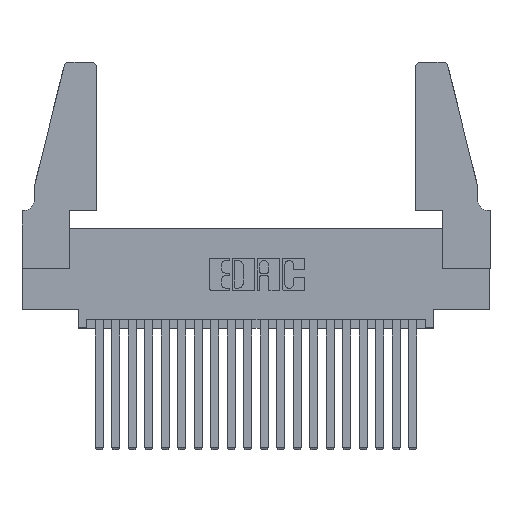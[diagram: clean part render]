
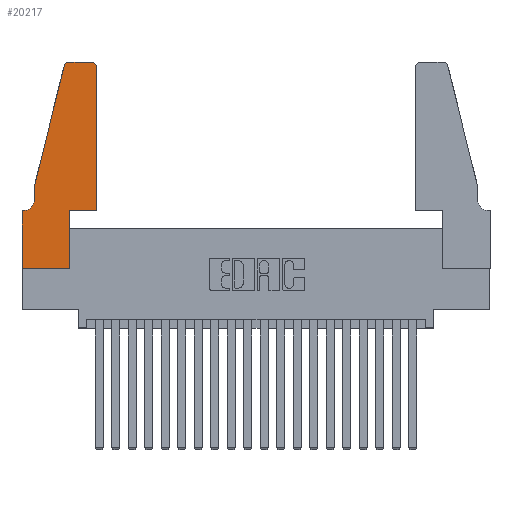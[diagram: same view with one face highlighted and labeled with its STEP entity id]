
A CAD part, top view. The second image highlights one B-rep face of the part: STEP entity #20217.
In plain terms, the highlighted planar face has unit normal (0, 0, 1).
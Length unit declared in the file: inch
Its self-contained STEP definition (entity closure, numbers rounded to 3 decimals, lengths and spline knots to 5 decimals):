
#63 = CIRCLE ( 'NONE', #4833, 0.03 ) ;
#71 = VECTOR ( 'NONE', #2145, 39.37008 ) ;
#83 = VECTOR ( 'NONE', #9493, 39.37008 ) ;
#277 = CARTESIAN_POINT ( 'NONE',  ( 0.2865, 0.35, 0.37 ) ) ;
#916 = ORIENTED_EDGE ( 'NONE', *, *, #2555, .T. ) ;
#964 = DIRECTION ( 'NONE',  ( 1., 0., 0. ) ) ;
#1077 = CARTESIAN_POINT ( 'NONE',  ( 0., 0., 0.37 ) ) ;
#1132 = EDGE_CURVE ( 'NONE', #18445, #18649, #6520, .T. ) ;
#1245 = CARTESIAN_POINT ( 'NONE',  ( 0.0755, 0.5, 0.37 ) ) ;
#1249 = VERTEX_POINT ( 'NONE', #6440 ) ;
#1459 = ORIENTED_EDGE ( 'NONE', *, *, #18032, .T. ) ;
#1578 = CIRCLE ( 'NONE', #18708, 0.03 ) ;
#1584 = CARTESIAN_POINT ( 'NONE',  ( 0., 0.35, 0.37 ) ) ;
#1736 = ORIENTED_EDGE ( 'NONE', *, *, #1132, .T. ) ;
#2145 = DIRECTION ( 'NONE',  ( 0., -1., 0. ) ) ;
#2345 = ORIENTED_EDGE ( 'NONE', *, *, #17151, .T. ) ;
#2362 = ORIENTED_EDGE ( 'NONE', *, *, #14664, .T. ) ;
#2456 = EDGE_CURVE ( 'NONE', #7041, #6586, #6937, .T. ) ;
#2555 = EDGE_CURVE ( 'NONE', #18649, #19597, #6683, .T. ) ;
#2651 = VERTEX_POINT ( 'NONE', #14811 ) ;
#3199 = CARTESIAN_POINT ( 'NONE',  ( 0.4205, 1.22, 0.37 ) ) ;
#3210 = DIRECTION ( 'NONE',  ( 0., 0., 1. ) ) ;
#3926 = EDGE_CURVE ( 'NONE', #1249, #4341, #18651, .T. ) ;
#4341 = VERTEX_POINT ( 'NONE', #12725 ) ;
#4622 = CARTESIAN_POINT ( 'NONE',  ( 0.2605, 1.25, 0.37 ) ) ;
#4833 = AXIS2_PLACEMENT_3D ( 'NONE', #5754, #20140, #964 ) ;
#5385 = ORIENTED_EDGE ( 'NONE', *, *, #16853, .T. ) ;
#5754 = CARTESIAN_POINT ( 'NONE',  ( 0.284, 1.22, 0.37 ) ) ;
#5901 = LINE ( 'NONE', #9222, #13915 ) ;
#6440 = CARTESIAN_POINT ( 'NONE',  ( 0.4205, 1.25, 0.37 ) ) ;
#6520 = LINE ( 'NONE', #1077, #14517 ) ;
#6586 = VERTEX_POINT ( 'NONE', #14233 ) ;
#6683 = LINE ( 'NONE', #9664, #11425 ) ;
#6937 = LINE ( 'NONE', #1245, #18170 ) ;
#6980 = EDGE_CURVE ( 'NONE', #19597, #17285, #10167, .T. ) ;
#7041 = VERTEX_POINT ( 'NONE', #12010 ) ;
#7139 = VECTOR ( 'NONE', #19183, 39.37008 ) ;
#7162 = LINE ( 'NONE', #14530, #8411 ) ;
#7263 = CARTESIAN_POINT ( 'NONE',  ( 0.4505, 0.35, 0.37 ) ) ;
#7593 = DIRECTION ( 'NONE',  ( -0.239, -0.971, 0. ) ) ;
#7916 = PLANE ( 'NONE',  #12781 ) ;
#7977 = EDGE_CURVE ( 'NONE', #9011, #1249, #1578, .T. ) ;
#7987 = CARTESIAN_POINT ( 'NONE',  ( 0.0055, 0.35, 0.37 ) ) ;
#8018 = ORIENTED_EDGE ( 'NONE', *, *, #17773, .T. ) ;
#8166 = DIRECTION ( 'NONE',  ( -1., 0., 0. ) ) ;
#8326 = AXIS2_PLACEMENT_3D ( 'NONE', #14010, #18814, #10862 ) ;
#8411 = VECTOR ( 'NONE', #8166, 39.37008 ) ;
#8809 = CARTESIAN_POINT ( 'NONE',  ( 0.4505, 0.35, 0.37 ) ) ;
#8859 = LINE ( 'NONE', #19618, #83 ) ;
#9011 = VERTEX_POINT ( 'NONE', #18805 ) ;
#9222 = CARTESIAN_POINT ( 'NONE',  ( 0.0755, 0.5, 0.37 ) ) ;
#9230 = ORIENTED_EDGE ( 'NONE', *, *, #7977, .T. ) ;
#9253 = ORIENTED_EDGE ( 'NONE', *, *, #2456, .T. ) ;
#9493 = DIRECTION ( 'NONE',  ( 0., 1., 0. ) ) ;
#9664 = CARTESIAN_POINT ( 'NONE',  ( 0.2865, 0.35, 0.37 ) ) ;
#10167 = LINE ( 'NONE', #8809, #11412 ) ;
#10442 = ORIENTED_EDGE ( 'NONE', *, *, #3926, .T. ) ;
#10549 = EDGE_LOOP ( 'NONE', ( #10442, #2345, #20662, #9253, #1459, #2362, #8018, #1736, #916, #19203, #5385, #9230 ) ) ;
#10594 = CARTESIAN_POINT ( 'NONE',  ( 0.25487, 1.22718, 0.37 ) ) ;
#10862 = DIRECTION ( 'NONE',  ( -1., 0., 0. ) ) ;
#11412 = VECTOR ( 'NONE', #13628, 39.37008 ) ;
#11425 = VECTOR ( 'NONE', #19174, 39.37008 ) ;
#12010 = CARTESIAN_POINT ( 'NONE',  ( 0.0755, 0.5, 0.37 ) ) ;
#12725 = CARTESIAN_POINT ( 'NONE',  ( 0.284, 1.25, 0.37 ) ) ;
#12781 = AXIS2_PLACEMENT_3D ( 'NONE', #1584, #3210, #14420 ) ;
#13628 = DIRECTION ( 'NONE',  ( 1., 0., 0. ) ) ;
#13915 = VECTOR ( 'NONE', #7593, 39.37008 ) ;
#14004 = VERTEX_POINT ( 'NONE', #7987 ) ;
#14010 = CARTESIAN_POINT ( 'NONE',  ( 0.0055, 0.42, 0.37 ) ) ;
#14073 = DIRECTION ( 'NONE',  ( 0., -1., 0. ) ) ;
#14119 = DIRECTION ( 'NONE',  ( 1., 0., 0. ) ) ;
#14233 = CARTESIAN_POINT ( 'NONE',  ( 0.0755, 0.42, 0.37 ) ) ;
#14420 = DIRECTION ( 'NONE',  ( 1., 0., 0. ) ) ;
#14502 = FACE_OUTER_BOUND ( 'NONE', #10549, .T. ) ;
#14517 = VECTOR ( 'NONE', #14119, 39.37008 ) ;
#14530 = CARTESIAN_POINT ( 'NONE',  ( 0.0755, 0.35, 0.37 ) ) ;
#14664 = EDGE_CURVE ( 'NONE', #14004, #2651, #7162, .T. ) ;
#14811 = CARTESIAN_POINT ( 'NONE',  ( 0., 0.35, 0.37 ) ) ;
#15195 = EDGE_CURVE ( 'NONE', #18552, #7041, #5901, .T. ) ;
#15507 = CARTESIAN_POINT ( 'NONE',  ( 0.2865, 0., 0.37 ) ) ;
#15870 = DIRECTION ( 'NONE',  ( 0., 0., 1. ) ) ;
#16853 = EDGE_CURVE ( 'NONE', #17285, #9011, #8859, .T. ) ;
#17151 = EDGE_CURVE ( 'NONE', #4341, #18552, #63, .T. ) ;
#17285 = VERTEX_POINT ( 'NONE', #7263 ) ;
#17587 = DIRECTION ( 'NONE',  ( 1., 0., 0. ) ) ;
#17696 = CARTESIAN_POINT ( 'NONE',  ( 0., 0., 0.37 ) ) ;
#17773 = EDGE_CURVE ( 'NONE', #2651, #18445, #18063, .T. ) ;
#18032 = EDGE_CURVE ( 'NONE', #6586, #14004, #18043, .T. ) ;
#18043 = CIRCLE ( 'NONE', #8326, 0.07 ) ;
#18063 = LINE ( 'NONE', #18831, #71 ) ;
#18170 = VECTOR ( 'NONE', #14073, 39.37008 ) ;
#18445 = VERTEX_POINT ( 'NONE', #17696 ) ;
#18552 = VERTEX_POINT ( 'NONE', #10594 ) ;
#18649 = VERTEX_POINT ( 'NONE', #15507 ) ;
#18651 = LINE ( 'NONE', #4622, #7139 ) ;
#18708 = AXIS2_PLACEMENT_3D ( 'NONE', #3199, #15870, #17587 ) ;
#18805 = CARTESIAN_POINT ( 'NONE',  ( 0.4505, 1.22, 0.37 ) ) ;
#18814 = DIRECTION ( 'NONE',  ( 0., 0., -1. ) ) ;
#18831 = CARTESIAN_POINT ( 'NONE',  ( 0., 0., 0.37 ) ) ;
#19174 = DIRECTION ( 'NONE',  ( 0., 1., 0. ) ) ;
#19183 = DIRECTION ( 'NONE',  ( -1., 0., 0. ) ) ;
#19203 = ORIENTED_EDGE ( 'NONE', *, *, #6980, .T. ) ;
#19597 = VERTEX_POINT ( 'NONE', #277 ) ;
#19618 = CARTESIAN_POINT ( 'NONE',  ( 0.4505, 0.35, 0.37 ) ) ;
#20140 = DIRECTION ( 'NONE',  ( 0., 0., 1. ) ) ;
#20217 = ADVANCED_FACE ( 'NONE', ( #14502 ), #7916, .T. ) ;
#20662 = ORIENTED_EDGE ( 'NONE', *, *, #15195, .T. ) ;
